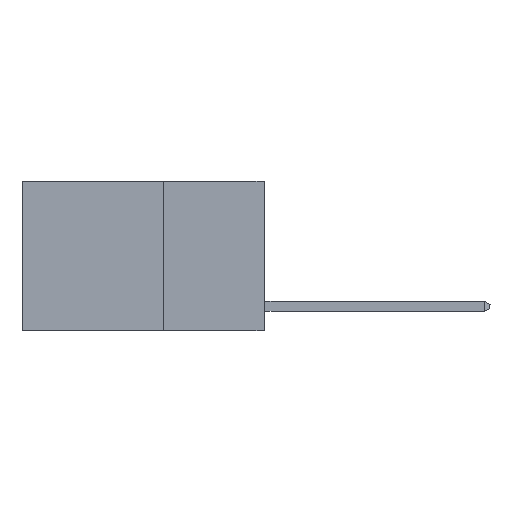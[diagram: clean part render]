
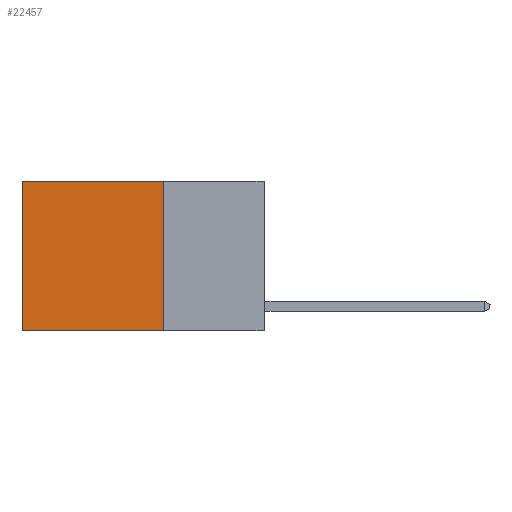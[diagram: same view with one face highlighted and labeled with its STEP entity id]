
A CAD part, left-side view. The second image highlights one B-rep face of the part: STEP entity #22457.
In plain terms, the highlighted planar face has unit normal (-1, 0, 0).
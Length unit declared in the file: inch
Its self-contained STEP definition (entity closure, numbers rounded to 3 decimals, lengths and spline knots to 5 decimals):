
#922 = VERTEX_POINT ( 'NONE', #5276 ) ;
#950 = PLANE ( 'NONE',  #23294 ) ;
#1661 = EDGE_CURVE ( 'NONE', #9408, #8012, #21444, .T. ) ;
#1833 = DIRECTION ( 'NONE',  ( 0., 1., 0. ) ) ;
#2524 = EDGE_CURVE ( 'NONE', #922, #6869, #21983, .T. ) ;
#2834 = CARTESIAN_POINT ( 'NONE',  ( 0.2625, 0.25, 0. ) ) ;
#3904 = CARTESIAN_POINT ( 'NONE',  ( 0.2625, 0.25, -0.37 ) ) ;
#4717 = DIRECTION ( 'NONE',  ( 1., 0., 0. ) ) ;
#5276 = CARTESIAN_POINT ( 'NONE',  ( 0.2625, 0.25, 0. ) ) ;
#5562 = FACE_OUTER_BOUND ( 'NONE', #21321, .T. ) ;
#5605 = CARTESIAN_POINT ( 'NONE',  ( 0.2625, 0.25, 0. ) ) ;
#5807 = DIRECTION ( 'NONE',  ( 0., 1., 0. ) ) ;
#5825 = ORIENTED_EDGE ( 'NONE', *, *, #1661, .T. ) ;
#6869 = VERTEX_POINT ( 'NONE', #22790 ) ;
#7086 = VECTOR ( 'NONE', #18264, 39.37008 ) ;
#8012 = VERTEX_POINT ( 'NONE', #20756 ) ;
#9408 = VERTEX_POINT ( 'NONE', #21808 ) ;
#11547 = VECTOR ( 'NONE', #21434, 39.37008 ) ;
#12968 = ORIENTED_EDGE ( 'NONE', *, *, #17993, .T. ) ;
#13383 = ORIENTED_EDGE ( 'NONE', *, *, #2524, .F. ) ;
#14824 = EDGE_CURVE ( 'NONE', #6869, #8012, #15719, .T. ) ;
#15719 = LINE ( 'NONE', #3904, #20123 ) ;
#16376 = CARTESIAN_POINT ( 'NONE',  ( 0.2625, 0.25, 0. ) ) ;
#17817 = DIRECTION ( 'NONE',  ( 0., 0., -1. ) ) ;
#17936 = LINE ( 'NONE', #5605, #21700 ) ;
#17993 = EDGE_CURVE ( 'NONE', #922, #9408, #17936, .T. ) ;
#18080 = CARTESIAN_POINT ( 'NONE',  ( 0.2625, 0.6, 0. ) ) ;
#18264 = DIRECTION ( 'NONE',  ( 0., 0., -1. ) ) ;
#20123 = VECTOR ( 'NONE', #5807, 39.37008 ) ;
#20756 = CARTESIAN_POINT ( 'NONE',  ( 0.2625, 0.6, -0.37 ) ) ;
#21321 = EDGE_LOOP ( 'NONE', ( #5825, #21341, #13383, #12968 ) ) ;
#21341 = ORIENTED_EDGE ( 'NONE', *, *, #14824, .F. ) ;
#21434 = DIRECTION ( 'NONE',  ( 0., 0., -1. ) ) ;
#21444 = LINE ( 'NONE', #18080, #11547 ) ;
#21700 = VECTOR ( 'NONE', #1833, 39.37008 ) ;
#21808 = CARTESIAN_POINT ( 'NONE',  ( 0.2625, 0.6, 0. ) ) ;
#21983 = LINE ( 'NONE', #16376, #7086 ) ;
#22457 = ADVANCED_FACE ( 'NONE', ( #5562 ), #950, .F. ) ;
#22790 = CARTESIAN_POINT ( 'NONE',  ( 0.2625, 0.25, -0.37 ) ) ;
#23294 = AXIS2_PLACEMENT_3D ( 'NONE', #2834, #4717, #17817 ) ;
